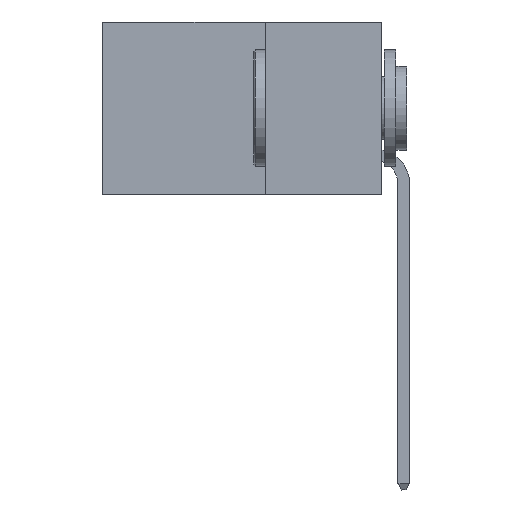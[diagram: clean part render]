
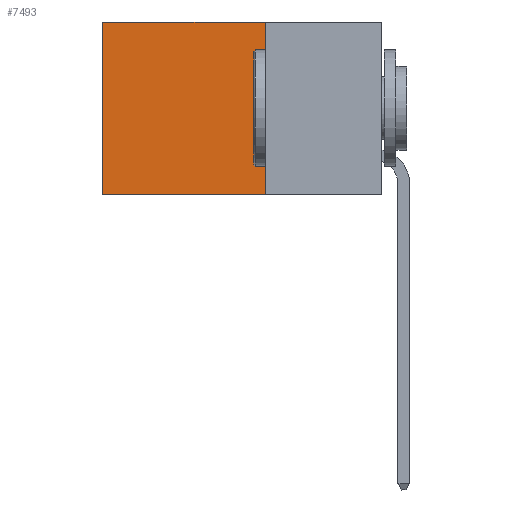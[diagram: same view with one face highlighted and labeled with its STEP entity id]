
A CAD part, left-side view. The second image highlights one B-rep face of the part: STEP entity #7493.
In plain terms, the highlighted planar face has unit normal (-1, 0, 0).
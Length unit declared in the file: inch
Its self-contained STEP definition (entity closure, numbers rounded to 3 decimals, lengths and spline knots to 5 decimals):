
#68 = CARTESIAN_POINT ( 'NONE',  ( 0.2875, 0.6, 0. ) ) ;
#968 = EDGE_CURVE ( 'NONE', #13641, #5857, #9463, .T. ) ;
#1052 = CARTESIAN_POINT ( 'NONE',  ( 0.2875, 0.6, 0. ) ) ;
#2059 = CARTESIAN_POINT ( 'NONE',  ( 0.2875, 0.25, 0. ) ) ;
#2543 = DIRECTION ( 'NONE',  ( 0., 0., -1. ) ) ;
#2749 = VECTOR ( 'NONE', #4337, 39.37008 ) ;
#3411 = DIRECTION ( 'NONE',  ( 1., 0., 0. ) ) ;
#3540 = EDGE_LOOP ( 'NONE', ( #15093, #13795, #7260, #10317 ) ) ;
#4337 = DIRECTION ( 'NONE',  ( 0., 1., 0. ) ) ;
#5857 = VERTEX_POINT ( 'NONE', #1052 ) ;
#6052 = VECTOR ( 'NONE', #2543, 39.37008 ) ;
#6067 = CARTESIAN_POINT ( 'NONE',  ( 0.2875, 0.6, -0.37 ) ) ;
#6433 = EDGE_CURVE ( 'NONE', #13641, #7842, #9472, .T. ) ;
#7241 = EDGE_CURVE ( 'NONE', #5857, #14546, #11464, .T. ) ;
#7260 = ORIENTED_EDGE ( 'NONE', *, *, #6433, .F. ) ;
#7493 = ADVANCED_FACE ( 'NONE', ( #11261 ), #9903, .F. ) ;
#7842 = VERTEX_POINT ( 'NONE', #10521 ) ;
#8503 = CARTESIAN_POINT ( 'NONE',  ( 0.2875, 0.25, 0. ) ) ;
#8757 = DIRECTION ( 'NONE',  ( 0., 1., 0. ) ) ;
#9463 = LINE ( 'NONE', #8503, #15879 ) ;
#9472 = LINE ( 'NONE', #12898, #6052 ) ;
#9536 = CARTESIAN_POINT ( 'NONE',  ( 0.2875, 0.25, 0. ) ) ;
#9903 = PLANE ( 'NONE',  #14949 ) ;
#10317 = ORIENTED_EDGE ( 'NONE', *, *, #968, .T. ) ;
#10521 = CARTESIAN_POINT ( 'NONE',  ( 0.2875, 0.25, -0.37 ) ) ;
#10654 = DIRECTION ( 'NONE',  ( 0., 0., -1. ) ) ;
#10814 = CARTESIAN_POINT ( 'NONE',  ( 0.2875, 0.25, -0.37 ) ) ;
#11261 = FACE_OUTER_BOUND ( 'NONE', #3540, .T. ) ;
#11464 = LINE ( 'NONE', #68, #11852 ) ;
#11852 = VECTOR ( 'NONE', #10654, 39.37008 ) ;
#12473 = DIRECTION ( 'NONE',  ( 0., 0., -1. ) ) ;
#12898 = CARTESIAN_POINT ( 'NONE',  ( 0.2875, 0.25, 0. ) ) ;
#13109 = EDGE_CURVE ( 'NONE', #7842, #14546, #13133, .T. ) ;
#13133 = LINE ( 'NONE', #10814, #2749 ) ;
#13641 = VERTEX_POINT ( 'NONE', #9536 ) ;
#13795 = ORIENTED_EDGE ( 'NONE', *, *, #13109, .F. ) ;
#14546 = VERTEX_POINT ( 'NONE', #6067 ) ;
#14949 = AXIS2_PLACEMENT_3D ( 'NONE', #2059, #3411, #12473 ) ;
#15093 = ORIENTED_EDGE ( 'NONE', *, *, #7241, .T. ) ;
#15879 = VECTOR ( 'NONE', #8757, 39.37008 ) ;
